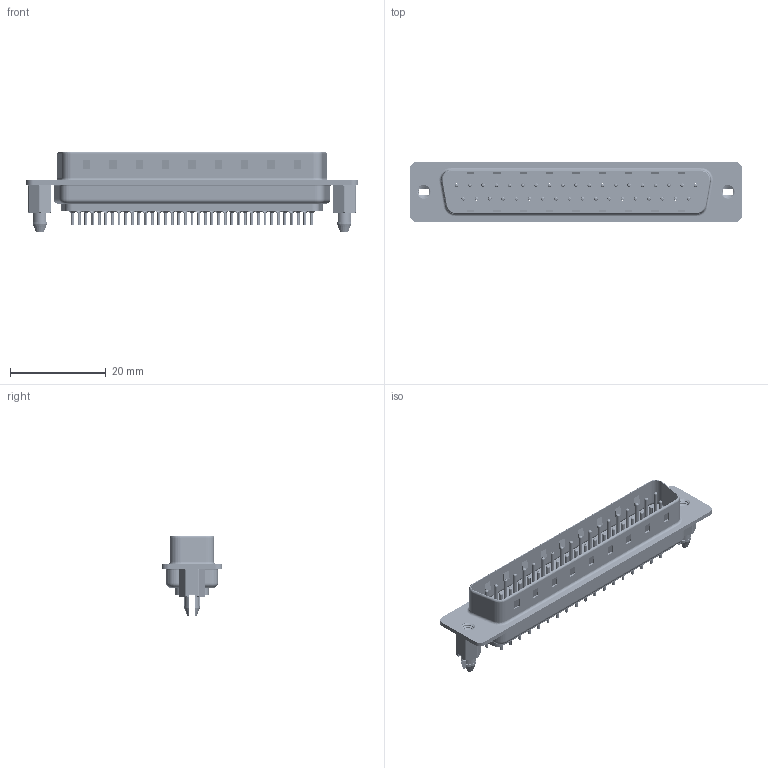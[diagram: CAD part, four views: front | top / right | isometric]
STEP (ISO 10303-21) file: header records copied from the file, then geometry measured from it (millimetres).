
FILE_DESCRIPTION (( 'STEP AP203' ), '1' );
FILE_NAME ('627-037-228-546.STEP', '2018-10-05T20:19:54', ( '' ), ( '' ), 'SwSTEP 2.0', 'SolidWorks 2016', '' );
FILE_SCHEMA (( 'CONFIG_CONTROL_DESIGN' ));
Length unit declared in the file: millimetre
Products named in the file (7): 627 Shell Rear_37 Contacts; 627 Contact Row 1_28L; 627 Contact Row 2_28L; 627 4-40 Threaded Boardlock_LP; 627-037-228-546; 627 Housing_37 LP; 627 Shell Front_37 Contacts
Assembly tree (42 placements, depth 2):
  627-037-228-546
    627 Housing_37 LP
    627 Shell Front_37 Contacts
    627 Shell Rear_37 Contacts
    627 Contact Row 1_28L  x19
    627 Contact Row 2_28L  x18
    627 4-40 Threaded Boardlock_LP  x2
Bounding box: 69.3 x 12.6 x 16.9 mm (x, y, z)
Volume: 3797.9 mm3; surface area: 10759.1 mm2
Topology: 42 solids, 42 shells, 4112 faces, 10800 edges, 6707 vertices
Faces by surface type: cylinder 1542, plane 1123, torus 1055, cone 386, bspline 6
Entity records: 30601 total; most frequent: CARTESIAN_POINT 6622, DIRECTION 4952, ORIENTED_EDGE 4458, EDGE_CURVE 2229, AXIS2_PLACEMENT_3D 1944, VERTEX_POINT 1431, EDGE_LOOP 1098, LINE 1064
